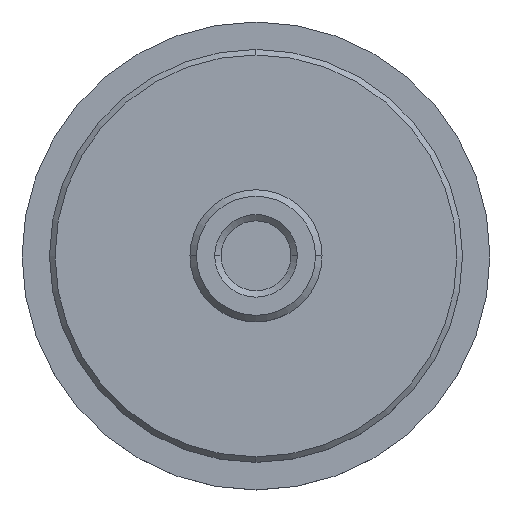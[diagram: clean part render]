
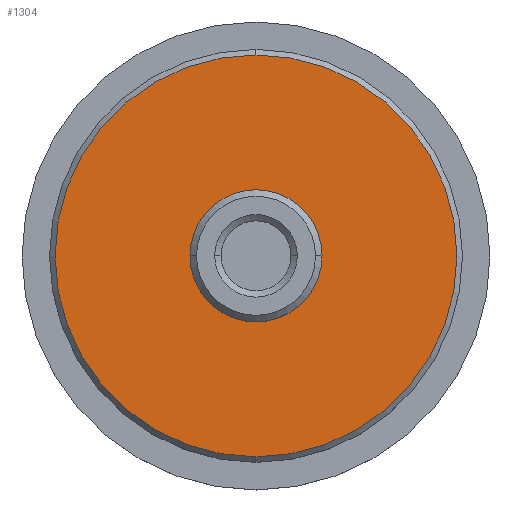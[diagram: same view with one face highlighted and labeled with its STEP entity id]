
A CAD part, top view. The second image highlights one B-rep face of the part: STEP entity #1304.
In plain terms, the highlighted planar face has unit normal (0, 0, 1).
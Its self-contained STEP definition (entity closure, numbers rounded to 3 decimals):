
#38 = DIRECTION ( 'NONE',  ( 0., 0., 1. ) ) ;
#48 = EDGE_CURVE ( 'NONE', #504, #1581, #343, .T. ) ;
#79 = ORIENTED_EDGE ( 'NONE', *, *, #587, .F. ) ;
#84 = DIRECTION ( 'NONE',  ( 1., 0., 0. ) ) ;
#114 = AXIS2_PLACEMENT_3D ( 'NONE', #749, #1328, #1660 ) ;
#172 = AXIS2_PLACEMENT_3D ( 'NONE', #519, #38, #84 ) ;
#233 = CARTESIAN_POINT ( 'NONE',  ( 0., 3.65, 0.15 ) ) ;
#261 = DIRECTION ( 'NONE',  ( 1., 0., 0. ) ) ;
#297 = AXIS2_PLACEMENT_3D ( 'NONE', #580, #1450, #444 ) ;
#332 = CIRCLE ( 'NONE', #1381, 1.2 ) ;
#343 = CIRCLE ( 'NONE', #1512, 3.65 ) ;
#353 = VERTEX_POINT ( 'NONE', #655 ) ;
#393 = CARTESIAN_POINT ( 'NONE',  ( 0., 0., 0.15 ) ) ;
#444 = DIRECTION ( 'NONE',  ( 1., 0., 0. ) ) ;
#469 = CARTESIAN_POINT ( 'NONE',  ( -1.2, 0., 0.15 ) ) ;
#478 = PLANE ( 'NONE',  #114 ) ;
#504 = VERTEX_POINT ( 'NONE', #1149 ) ;
#509 = FACE_BOUND ( 'NONE', #1640, .T. ) ;
#519 = CARTESIAN_POINT ( 'NONE',  ( 0., 0., 0.15 ) ) ;
#554 = DIRECTION ( 'NONE',  ( 0., 0., 1. ) ) ;
#580 = CARTESIAN_POINT ( 'NONE',  ( 0., 0., 0.15 ) ) ;
#587 = EDGE_CURVE ( 'NONE', #625, #353, #1193, .T. ) ;
#625 = VERTEX_POINT ( 'NONE', #469 ) ;
#655 = CARTESIAN_POINT ( 'NONE',  ( 1.2, 0., 0.15 ) ) ;
#749 = CARTESIAN_POINT ( 'NONE',  ( 0., 0., 0.15 ) ) ;
#779 = EDGE_CURVE ( 'NONE', #1581, #504, #1318, .T. ) ;
#834 = CARTESIAN_POINT ( 'NONE',  ( 0., 0., 0.15 ) ) ;
#1143 = ORIENTED_EDGE ( 'NONE', *, *, #779, .T. ) ;
#1149 = CARTESIAN_POINT ( 'NONE',  ( 0., -3.65, 0.15 ) ) ;
#1193 = CIRCLE ( 'NONE', #297, 1.2 ) ;
#1195 = EDGE_CURVE ( 'NONE', #353, #625, #332, .T. ) ;
#1304 = ADVANCED_FACE ( 'NONE', ( #509, #1613 ), #478, .T. ) ;
#1318 = CIRCLE ( 'NONE', #172, 3.65 ) ;
#1328 = DIRECTION ( 'NONE',  ( 0., 0., 1. ) ) ;
#1363 = ORIENTED_EDGE ( 'NONE', *, *, #1195, .F. ) ;
#1381 = AXIS2_PLACEMENT_3D ( 'NONE', #834, #554, #1418 ) ;
#1418 = DIRECTION ( 'NONE',  ( 1., 0., 0. ) ) ;
#1450 = DIRECTION ( 'NONE',  ( 0., 0., 1. ) ) ;
#1512 = AXIS2_PLACEMENT_3D ( 'NONE', #393, #1537, #261 ) ;
#1537 = DIRECTION ( 'NONE',  ( 0., 0., 1. ) ) ;
#1581 = VERTEX_POINT ( 'NONE', #233 ) ;
#1613 = FACE_OUTER_BOUND ( 'NONE', #1750, .T. ) ;
#1640 = EDGE_LOOP ( 'NONE', ( #79, #1363 ) ) ;
#1660 = DIRECTION ( 'NONE',  ( 1., 0., 0. ) ) ;
#1750 = EDGE_LOOP ( 'NONE', ( #1770, #1143 ) ) ;
#1770 = ORIENTED_EDGE ( 'NONE', *, *, #48, .T. ) ;
